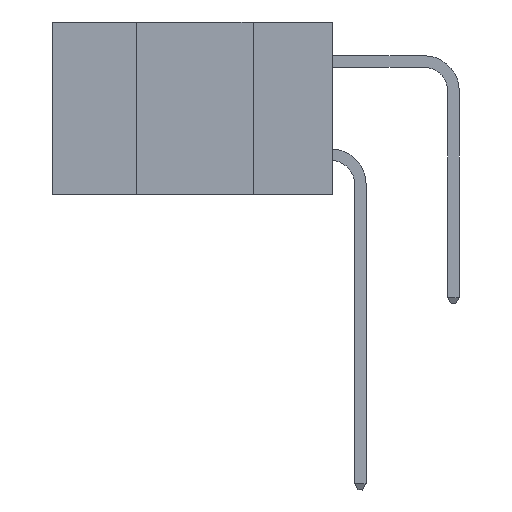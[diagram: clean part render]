
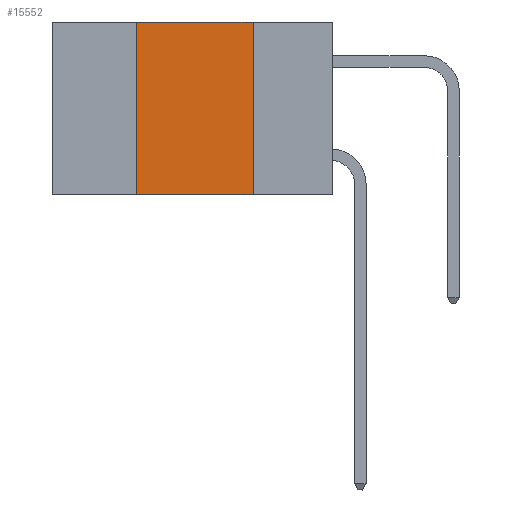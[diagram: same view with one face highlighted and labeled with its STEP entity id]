
A CAD part, left-side view. The second image highlights one B-rep face of the part: STEP entity #15552.
In plain terms, the highlighted planar face has unit normal (-1, 0, 0).
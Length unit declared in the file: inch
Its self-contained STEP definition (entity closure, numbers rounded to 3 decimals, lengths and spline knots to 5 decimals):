
#109 = CARTESIAN_POINT ( 'NONE',  ( 0., 0.6, 0. ) ) ;
#299 = EDGE_LOOP ( 'NONE', ( #13538, #2438, #1992, #19494 ) ) ;
#660 = LINE ( 'NONE', #16268, #18974 ) ;
#756 = CARTESIAN_POINT ( 'NONE',  ( 0., 0.17, 0. ) ) ;
#1086 = EDGE_CURVE ( 'NONE', #13617, #21611, #21783, .T. ) ;
#1098 = DIRECTION ( 'NONE',  ( 0., 0., 1. ) ) ;
#1203 = VERTEX_POINT ( 'NONE', #756 ) ;
#1992 = ORIENTED_EDGE ( 'NONE', *, *, #1086, .F. ) ;
#2038 = DIRECTION ( 'NONE',  ( 1., 0., 0. ) ) ;
#2438 = ORIENTED_EDGE ( 'NONE', *, *, #16584, .F. ) ;
#2549 = EDGE_CURVE ( 'NONE', #1203, #17913, #660, .T. ) ;
#5027 = LINE ( 'NONE', #11956, #22032 ) ;
#5138 = VECTOR ( 'NONE', #1098, 39.37008 ) ;
#7193 = CARTESIAN_POINT ( 'NONE',  ( 0., 0.6, -0.37 ) ) ;
#7528 = DIRECTION ( 'NONE',  ( 0., 0., -1. ) ) ;
#8808 = DIRECTION ( 'NONE',  ( 0., -1., 0. ) ) ;
#8870 = DIRECTION ( 'NONE',  ( 0., -1., 0. ) ) ;
#9344 = CARTESIAN_POINT ( 'NONE',  ( 0., 0.42, 0. ) ) ;
#10538 = LINE ( 'NONE', #7193, #13698 ) ;
#11820 = CARTESIAN_POINT ( 'NONE',  ( 0., 0.42, -0.37 ) ) ;
#11956 = CARTESIAN_POINT ( 'NONE',  ( 0., 0.6, 0. ) ) ;
#12331 = PLANE ( 'NONE',  #14156 ) ;
#12907 = EDGE_CURVE ( 'NONE', #13617, #17913, #10538, .T. ) ;
#13538 = ORIENTED_EDGE ( 'NONE', *, *, #2549, .F. ) ;
#13617 = VERTEX_POINT ( 'NONE', #11820 ) ;
#13698 = VECTOR ( 'NONE', #8808, 39.37008 ) ;
#14156 = AXIS2_PLACEMENT_3D ( 'NONE', #109, #2038, #17510 ) ;
#14161 = FACE_OUTER_BOUND ( 'NONE', #299, .T. ) ;
#15552 = ADVANCED_FACE ( 'NONE', ( #14161 ), #12331, .F. ) ;
#16268 = CARTESIAN_POINT ( 'NONE',  ( 0., 0.17, -0.37 ) ) ;
#16584 = EDGE_CURVE ( 'NONE', #21611, #1203, #5027, .T. ) ;
#17256 = CARTESIAN_POINT ( 'NONE',  ( 0., 0.17, -0.37 ) ) ;
#17510 = DIRECTION ( 'NONE',  ( 0., 0., -1. ) ) ;
#17913 = VERTEX_POINT ( 'NONE', #17256 ) ;
#18974 = VECTOR ( 'NONE', #7528, 39.37008 ) ;
#19494 = ORIENTED_EDGE ( 'NONE', *, *, #12907, .T. ) ;
#19966 = CARTESIAN_POINT ( 'NONE',  ( 0., 0.42, -0.37 ) ) ;
#21611 = VERTEX_POINT ( 'NONE', #9344 ) ;
#21783 = LINE ( 'NONE', #19966, #5138 ) ;
#22032 = VECTOR ( 'NONE', #8870, 39.37008 ) ;
